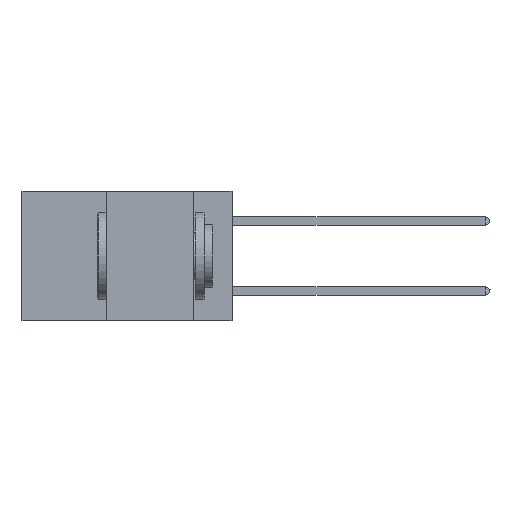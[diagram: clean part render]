
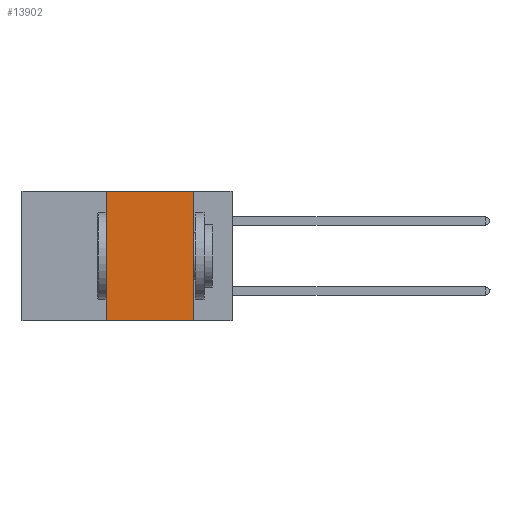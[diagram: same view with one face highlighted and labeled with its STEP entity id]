
A CAD part, left-side view. The second image highlights one B-rep face of the part: STEP entity #13902.
In plain terms, the highlighted planar face has unit normal (-1, 0, 0).
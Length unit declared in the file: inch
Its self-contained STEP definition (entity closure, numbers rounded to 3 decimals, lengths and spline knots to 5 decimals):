
#233 = CARTESIAN_POINT ( 'NONE',  ( 0., 0.6, 0. ) ) ;
#280 = DIRECTION ( 'NONE',  ( 1., 0., 0. ) ) ;
#518 = CARTESIAN_POINT ( 'NONE',  ( 0., 0.36, 0. ) ) ;
#1069 = CARTESIAN_POINT ( 'NONE',  ( 0., 0.11, 0. ) ) ;
#2139 = DIRECTION ( 'NONE',  ( 0., -1., 0. ) ) ;
#2378 = VERTEX_POINT ( 'NONE', #8934 ) ;
#3073 = ORIENTED_EDGE ( 'NONE', *, *, #7440, .F. ) ;
#3357 = CARTESIAN_POINT ( 'NONE',  ( 0., 0.36, -0.37 ) ) ;
#3951 = DIRECTION ( 'NONE',  ( 0., 0., -1. ) ) ;
#3982 = EDGE_LOOP ( 'NONE', ( #3073, #8291, #24027, #8116 ) ) ;
#4120 = PLANE ( 'NONE',  #15616 ) ;
#4343 = LINE ( 'NONE', #18896, #17767 ) ;
#5695 = LINE ( 'NONE', #233, #15221 ) ;
#7193 = EDGE_CURVE ( 'NONE', #11443, #17826, #15270, .T. ) ;
#7440 = EDGE_CURVE ( 'NONE', #20966, #2378, #22988, .T. ) ;
#8116 = ORIENTED_EDGE ( 'NONE', *, *, #15021, .T. ) ;
#8291 = ORIENTED_EDGE ( 'NONE', *, *, #18544, .F. ) ;
#8934 = CARTESIAN_POINT ( 'NONE',  ( 0., 0.11, -0.37 ) ) ;
#9467 = FACE_OUTER_BOUND ( 'NONE', #3982, .T. ) ;
#9584 = CARTESIAN_POINT ( 'NONE',  ( 0., 0.36, 0. ) ) ;
#10579 = DIRECTION ( 'NONE',  ( 0., 0., -1. ) ) ;
#11067 = VECTOR ( 'NONE', #19338, 39.37008 ) ;
#11443 = VERTEX_POINT ( 'NONE', #3357 ) ;
#13782 = VECTOR ( 'NONE', #10579, 39.37008 ) ;
#13902 = ADVANCED_FACE ( 'NONE', ( #9467 ), #4120, .F. ) ;
#15021 = EDGE_CURVE ( 'NONE', #11443, #2378, #4343, .T. ) ;
#15221 = VECTOR ( 'NONE', #2139, 39.37008 ) ;
#15270 = LINE ( 'NONE', #518, #11067 ) ;
#15616 = AXIS2_PLACEMENT_3D ( 'NONE', #17645, #280, #3951 ) ;
#16827 = DIRECTION ( 'NONE',  ( 0., -1., 0. ) ) ;
#16884 = CARTESIAN_POINT ( 'NONE',  ( 0., 0.11, 0. ) ) ;
#17645 = CARTESIAN_POINT ( 'NONE',  ( 0., 0.6, 0. ) ) ;
#17767 = VECTOR ( 'NONE', #16827, 39.37008 ) ;
#17826 = VERTEX_POINT ( 'NONE', #9584 ) ;
#18544 = EDGE_CURVE ( 'NONE', #17826, #20966, #5695, .T. ) ;
#18896 = CARTESIAN_POINT ( 'NONE',  ( 0., 0.6, -0.37 ) ) ;
#19338 = DIRECTION ( 'NONE',  ( 0., 0., 1. ) ) ;
#20966 = VERTEX_POINT ( 'NONE', #16884 ) ;
#22988 = LINE ( 'NONE', #1069, #13782 ) ;
#24027 = ORIENTED_EDGE ( 'NONE', *, *, #7193, .F. ) ;
